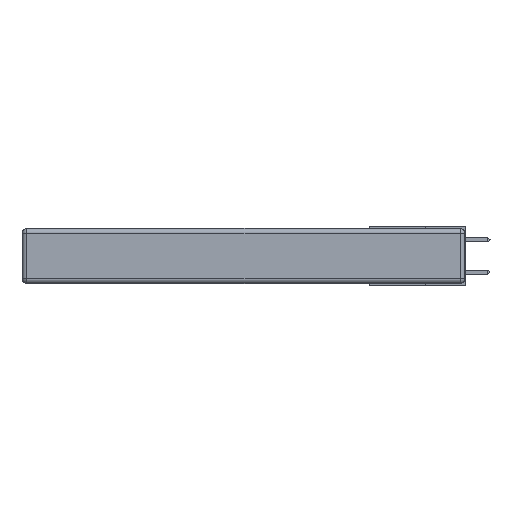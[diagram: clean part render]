
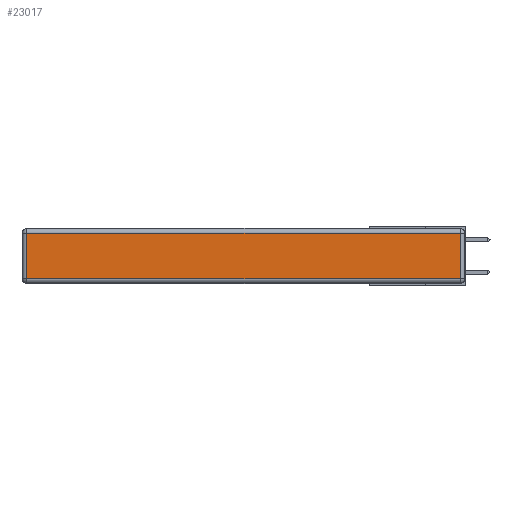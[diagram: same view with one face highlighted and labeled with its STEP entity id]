
A CAD part, left-side view. The second image highlights one B-rep face of the part: STEP entity #23017.
In plain terms, the highlighted planar face has unit normal (-1, 0, 0).
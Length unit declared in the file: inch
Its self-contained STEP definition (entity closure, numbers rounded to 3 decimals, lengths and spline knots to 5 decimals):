
#20 = CARTESIAN_POINT ( 'NONE',  ( 0., 0.03, -0.03 ) ) ;
#364 = CARTESIAN_POINT ( 'NONE',  ( 0., 2.75, -0.03 ) ) ;
#1310 = CARTESIAN_POINT ( 'NONE',  ( 0., 2.72, -0.343 ) ) ;
#1892 = LINE ( 'NONE', #18796, #11695 ) ;
#2510 = LINE ( 'NONE', #13020, #4430 ) ;
#3331 = VERTEX_POINT ( 'NONE', #20 ) ;
#3628 = CARTESIAN_POINT ( 'NONE',  ( 0., 0., -0.343 ) ) ;
#3723 = ORIENTED_EDGE ( 'NONE', *, *, #13168, .T. ) ;
#3724 = LINE ( 'NONE', #364, #12582 ) ;
#4430 = VECTOR ( 'NONE', #25350, 39.37008 ) ;
#5720 = DIRECTION ( 'NONE',  ( 0., 0., 1. ) ) ;
#5932 = FACE_OUTER_BOUND ( 'NONE', #14132, .T. ) ;
#6992 = AXIS2_PLACEMENT_3D ( 'NONE', #3628, #18213, #5720 ) ;
#8195 = ORIENTED_EDGE ( 'NONE', *, *, #10376, .T. ) ;
#8901 = CARTESIAN_POINT ( 'NONE',  ( 0., 2.72, -0.03 ) ) ;
#9442 = LINE ( 'NONE', #1310, #18838 ) ;
#10376 = EDGE_CURVE ( 'NONE', #16085, #19272, #9442, .T. ) ;
#11032 = ORIENTED_EDGE ( 'NONE', *, *, #25737, .T. ) ;
#11695 = VECTOR ( 'NONE', #12422, 39.37008 ) ;
#11713 = EDGE_CURVE ( 'NONE', #21144, #3331, #2510, .T. ) ;
#12422 = DIRECTION ( 'NONE',  ( 0., -1., 0. ) ) ;
#12582 = VECTOR ( 'NONE', #18901, 39.37008 ) ;
#13020 = CARTESIAN_POINT ( 'NONE',  ( 0., 0.03, -0.343 ) ) ;
#13075 = CARTESIAN_POINT ( 'NONE',  ( 0., 2.72, -0.313 ) ) ;
#13168 = EDGE_CURVE ( 'NONE', #3331, #16085, #3724, .T. ) ;
#14132 = EDGE_LOOP ( 'NONE', ( #11032, #19737, #3723, #8195 ) ) ;
#15866 = DIRECTION ( 'NONE',  ( 0., 0., -1. ) ) ;
#16085 = VERTEX_POINT ( 'NONE', #8901 ) ;
#18213 = DIRECTION ( 'NONE',  ( -1., 0., 0. ) ) ;
#18297 = CARTESIAN_POINT ( 'NONE',  ( 0., 0.03, -0.313 ) ) ;
#18796 = CARTESIAN_POINT ( 'NONE',  ( 0., 0., -0.313 ) ) ;
#18838 = VECTOR ( 'NONE', #15866, 39.37008 ) ;
#18901 = DIRECTION ( 'NONE',  ( 0., 1., 0. ) ) ;
#19272 = VERTEX_POINT ( 'NONE', #13075 ) ;
#19737 = ORIENTED_EDGE ( 'NONE', *, *, #11713, .T. ) ;
#21144 = VERTEX_POINT ( 'NONE', #18297 ) ;
#22128 = PLANE ( 'NONE',  #6992 ) ;
#23017 = ADVANCED_FACE ( 'NONE', ( #5932 ), #22128, .T. ) ;
#25350 = DIRECTION ( 'NONE',  ( 0., 0., 1. ) ) ;
#25737 = EDGE_CURVE ( 'NONE', #19272, #21144, #1892, .T. ) ;
